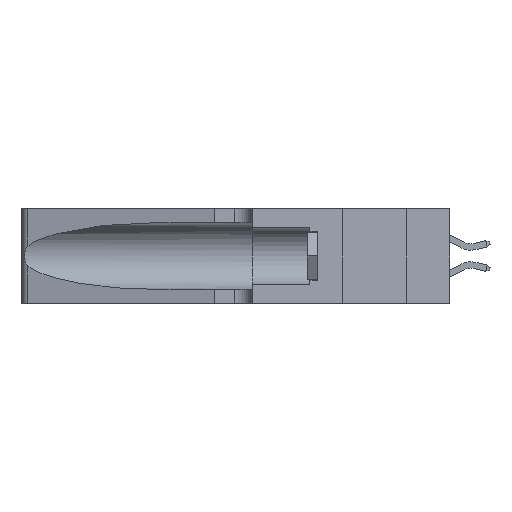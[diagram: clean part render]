
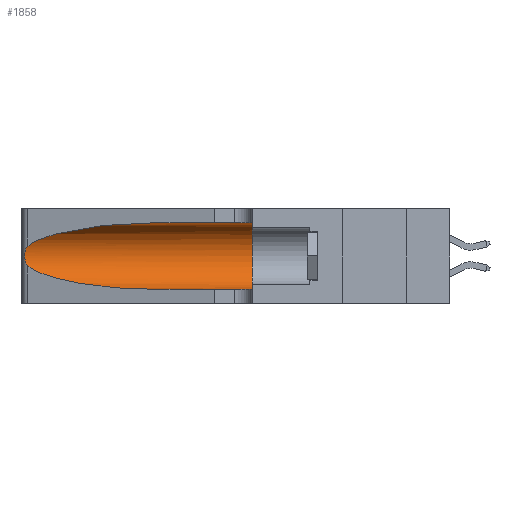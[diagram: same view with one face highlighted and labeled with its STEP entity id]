
A CAD part, left-side view. The second image highlights one B-rep face of the part: STEP entity #1858.
In plain terms, the highlighted cylindrical face has radius 3.308 mm (diameter 6.617 mm), a partial arc.
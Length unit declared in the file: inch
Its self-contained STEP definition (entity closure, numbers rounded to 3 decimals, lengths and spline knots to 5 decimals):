
#341 = DIRECTION ( 'NONE',  ( 0., 0., -1. ) ) ;
#386 = VERTEX_POINT ( 'NONE', #4901 ) ;
#439 = CARTESIAN_POINT ( 'NONE',  ( 0.26075, 1.23896, 0.178 ) ) ;
#765 = CARTESIAN_POINT ( 'NONE',  ( 0.1305, 0.35, 0.185 ) ) ;
#951 = DIRECTION ( 'NONE',  ( 0., 0., 1. ) ) ;
#1312 = CARTESIAN_POINT ( 'NONE',  ( 0.25487, 1.22718, 0.22369 ) ) ;
#1509 =( BOUNDED_CURVE ( )  B_SPLINE_CURVE ( 3, ( #7896, #17220, #11102, #1312 ),
 .UNSPECIFIED., .F., .F. ) 
 B_SPLINE_CURVE_WITH_KNOTS ( ( 4, 4 ),
 ( 1.5708, 2.84003 ),
 .UNSPECIFIED. ) 
 CURVE ( )  GEOMETRIC_REPRESENTATION_ITEM ( )  RATIONAL_B_SPLINE_CURVE ( ( 1., 0.87, 0.87, 1. ) ) 
 REPRESENTATION_ITEM ( '' )  );
#1858 = ADVANCED_FACE ( 'NONE', ( #3986 ), #15661, .F. ) ;
#2193 = B_SPLINE_CURVE_WITH_KNOTS ( 'NONE', 3,
 ( #5401, #16435, #7057, #17958, #8685, #19469, #10310, #439, #11842, #5617, #5374, #8061, #18882, #9675 ),
 .UNSPECIFIED., .F., .F.,
 ( 4, 2, 2, 2, 2, 2, 4 ),
 ( 0., 0.00027, 0.00053, 0.00107, 0.0016, 0.00187, 0.00214 ),
 .UNSPECIFIED. ) ;
#2555 = CARTESIAN_POINT ( 'NONE',  ( 0.1305, 0.72297, 0.05475 ) ) ;
#2593 =( BOUNDED_CURVE ( )  B_SPLINE_CURVE ( 3, ( #9327, #14043, #7773, #18620 ),
 .UNSPECIFIED., .F., .F. ) 
 B_SPLINE_CURVE_WITH_KNOTS ( ( 4, 4 ),
 ( 3.44316, 4.71239 ),
 .UNSPECIFIED. ) 
 CURVE ( )  GEOMETRIC_REPRESENTATION_ITEM ( )  RATIONAL_B_SPLINE_CURVE ( ( 1., 0.87, 0.87, 1. ) ) 
 REPRESENTATION_ITEM ( '' )  );
#2689 = VERTEX_POINT ( 'NONE', #3729 ) ;
#2992 = VERTEX_POINT ( 'NONE', #2555 ) ;
#3402 = EDGE_CURVE ( 'NONE', #6998, #17230, #7062, .T. ) ;
#3729 = CARTESIAN_POINT ( 'NONE',  ( 0.25487, 1.22718, 0.14631 ) ) ;
#3986 = FACE_OUTER_BOUND ( 'NONE', #4610, .T. ) ;
#4445 = DIRECTION ( 'NONE',  ( 0., -1., 0. ) ) ;
#4610 = EDGE_LOOP ( 'NONE', ( #8573, #5094, #17134, #11029, #12698, #11725 ) ) ;
#4901 = CARTESIAN_POINT ( 'NONE',  ( 0.1305, 0.72297, 0.31525 ) ) ;
#4950 = LINE ( 'NONE', #15541, #17030 ) ;
#5094 = ORIENTED_EDGE ( 'NONE', *, *, #6888, .T. ) ;
#5374 = CARTESIAN_POINT ( 'NONE',  ( 0.25789, 1.23486, 0.15765 ) ) ;
#5384 = CARTESIAN_POINT ( 'NONE',  ( 0.1305, 1.61858, 0.185 ) ) ;
#5401 = CARTESIAN_POINT ( 'NONE',  ( 0.25487, 1.22718, 0.22369 ) ) ;
#5617 = CARTESIAN_POINT ( 'NONE',  ( 0.25856, 1.23593, 0.16098 ) ) ;
#5739 = CARTESIAN_POINT ( 'NONE',  ( 0.1305, 0.35, 0.05475 ) ) ;
#6294 = DIRECTION ( 'NONE',  ( 0., -1., 0. ) ) ;
#6542 = EDGE_CURVE ( 'NONE', #2689, #2992, #2593, .T. ) ;
#6888 = EDGE_CURVE ( 'NONE', #18452, #2689, #2193, .T. ) ;
#6998 = VERTEX_POINT ( 'NONE', #14579 ) ;
#7057 = CARTESIAN_POINT ( 'NONE',  ( 0.25639, 1.23184, 0.21858 ) ) ;
#7062 = CIRCLE ( 'NONE', #14760, 0.13025 ) ;
#7318 = DIRECTION ( 'NONE',  ( 0., 1., 0. ) ) ;
#7773 = CARTESIAN_POINT ( 'NONE',  ( 0.18966, 0.96281, 0.05475 ) ) ;
#7896 = CARTESIAN_POINT ( 'NONE',  ( 0.1305, 0.72297, 0.31525 ) ) ;
#8061 = CARTESIAN_POINT ( 'NONE',  ( 0.25639, 1.23186, 0.15144 ) ) ;
#8573 = ORIENTED_EDGE ( 'NONE', *, *, #9419, .T. ) ;
#8685 = CARTESIAN_POINT ( 'NONE',  ( 0.25854, 1.2359, 0.20912 ) ) ;
#9327 = CARTESIAN_POINT ( 'NONE',  ( 0.25487, 1.22718, 0.14631 ) ) ;
#9419 = EDGE_CURVE ( 'NONE', #386, #18452, #1509, .T. ) ;
#9675 = CARTESIAN_POINT ( 'NONE',  ( 0.25487, 1.22718, 0.14631 ) ) ;
#9988 = LINE ( 'NONE', #20283, #17698 ) ;
#10310 = CARTESIAN_POINT ( 'NONE',  ( 0.26075, 1.23896, 0.19203 ) ) ;
#10519 = CARTESIAN_POINT ( 'NONE',  ( 0.25487, 1.22718, 0.22369 ) ) ;
#11029 = ORIENTED_EDGE ( 'NONE', *, *, #13803, .T. ) ;
#11102 = CARTESIAN_POINT ( 'NONE',  ( 0.2373, 1.15595, 0.28018 ) ) ;
#11725 = ORIENTED_EDGE ( 'NONE', *, *, #19417, .F. ) ;
#11842 = CARTESIAN_POINT ( 'NONE',  ( 0.26017, 1.23833, 0.17102 ) ) ;
#12698 = ORIENTED_EDGE ( 'NONE', *, *, #3402, .F. ) ;
#13184 = AXIS2_PLACEMENT_3D ( 'NONE', #5384, #16267, #341 ) ;
#13803 = EDGE_CURVE ( 'NONE', #2992, #17230, #9988, .T. ) ;
#14043 = CARTESIAN_POINT ( 'NONE',  ( 0.2373, 1.15595, 0.08982 ) ) ;
#14579 = CARTESIAN_POINT ( 'NONE',  ( 0.1305, 0.35, 0.31525 ) ) ;
#14760 = AXIS2_PLACEMENT_3D ( 'NONE', #765, #7318, #951 ) ;
#15541 = CARTESIAN_POINT ( 'NONE',  ( 0.1305, 1.61858, 0.31525 ) ) ;
#15661 = CYLINDRICAL_SURFACE ( 'NONE', #13184, 0.13025 ) ;
#16267 = DIRECTION ( 'NONE',  ( 0., -1., 0. ) ) ;
#16435 = CARTESIAN_POINT ( 'NONE',  ( 0.25555, 1.22994, 0.2215 ) ) ;
#17030 = VECTOR ( 'NONE', #4445, 39.37008 ) ;
#17134 = ORIENTED_EDGE ( 'NONE', *, *, #6542, .T. ) ;
#17220 = CARTESIAN_POINT ( 'NONE',  ( 0.18966, 0.96281, 0.31525 ) ) ;
#17230 = VERTEX_POINT ( 'NONE', #5739 ) ;
#17698 = VECTOR ( 'NONE', #6294, 39.37008 ) ;
#17958 = CARTESIAN_POINT ( 'NONE',  ( 0.25787, 1.23484, 0.2124 ) ) ;
#18452 = VERTEX_POINT ( 'NONE', #10519 ) ;
#18620 = CARTESIAN_POINT ( 'NONE',  ( 0.1305, 0.72297, 0.05475 ) ) ;
#18882 = CARTESIAN_POINT ( 'NONE',  ( 0.25555, 1.22993, 0.14849 ) ) ;
#19417 = EDGE_CURVE ( 'NONE', #386, #6998, #4950, .T. ) ;
#19469 = CARTESIAN_POINT ( 'NONE',  ( 0.26018, 1.23835, 0.19895 ) ) ;
#20283 = CARTESIAN_POINT ( 'NONE',  ( 0.1305, 1.61858, 0.05475 ) ) ;
